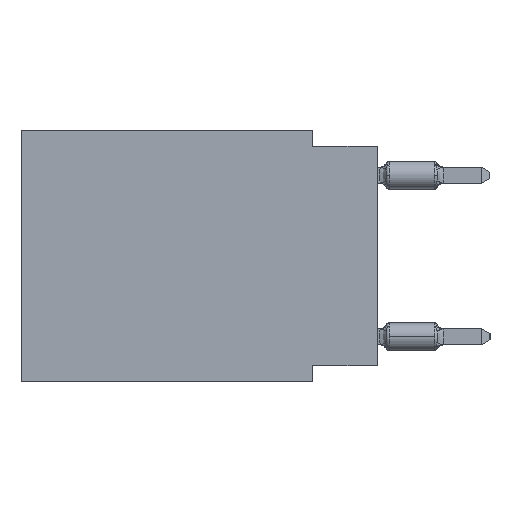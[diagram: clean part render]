
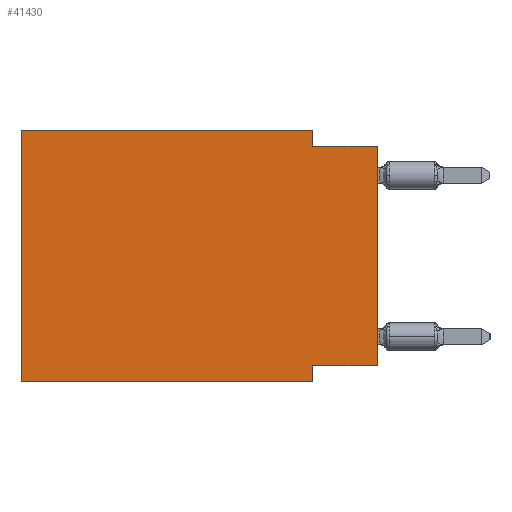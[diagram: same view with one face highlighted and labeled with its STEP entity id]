
A CAD part, left-side view. The second image highlights one B-rep face of the part: STEP entity #41430.
In plain terms, the highlighted planar face has unit normal (-1, 0, 0).
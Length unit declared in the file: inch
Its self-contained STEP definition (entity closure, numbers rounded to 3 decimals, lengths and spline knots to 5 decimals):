
#251 = EDGE_CURVE ( 'NONE', #14994, #14648, #38227, .T. ) ;
#1820 = EDGE_CURVE ( 'NONE', #37931, #29589, #4543, .T. ) ;
#2186 = DIRECTION ( 'NONE',  ( 0., 0., 1. ) ) ;
#2414 = CARTESIAN_POINT ( 'NONE',  ( 0., 0., 0. ) ) ;
#3234 = CARTESIAN_POINT ( 'NONE',  ( 0., 0.55, -0.39 ) ) ;
#4543 = LINE ( 'NONE', #5218, #20845 ) ;
#5218 = CARTESIAN_POINT ( 'NONE',  ( 0., 0.1, 0. ) ) ;
#6077 = DIRECTION ( 'NONE',  ( 0., 0., -1. ) ) ;
#8016 = ORIENTED_EDGE ( 'NONE', *, *, #33502, .T. ) ;
#8417 = CARTESIAN_POINT ( 'NONE',  ( 0., 0.1, -0.365 ) ) ;
#10371 = VERTEX_POINT ( 'NONE', #8417 ) ;
#11001 = ORIENTED_EDGE ( 'NONE', *, *, #20388, .F. ) ;
#11477 = VECTOR ( 'NONE', #44151, 39.37008 ) ;
#11637 = DIRECTION ( 'NONE',  ( 0., 0., -1. ) ) ;
#11897 = EDGE_LOOP ( 'NONE', ( #8016, #33574, #43823, #37226, #11001, #32263, #31227, #36981 ) ) ;
#12938 = CARTESIAN_POINT ( 'NONE',  ( 0., 0.1, -0.39 ) ) ;
#14648 = VERTEX_POINT ( 'NONE', #43078 ) ;
#14994 = VERTEX_POINT ( 'NONE', #20592 ) ;
#15985 = VECTOR ( 'NONE', #43843, 39.37008 ) ;
#16177 = CARTESIAN_POINT ( 'NONE',  ( 0., 0.1, -0.025 ) ) ;
#16811 = FACE_OUTER_BOUND ( 'NONE', #11897, .T. ) ;
#17160 = DIRECTION ( 'NONE',  ( 0., -1., 0. ) ) ;
#17559 = LINE ( 'NONE', #31271, #32658 ) ;
#17664 = CARTESIAN_POINT ( 'NONE',  ( 0., 0., -0.365 ) ) ;
#20088 = EDGE_CURVE ( 'NONE', #29589, #35310, #26798, .T. ) ;
#20388 = EDGE_CURVE ( 'NONE', #14994, #23673, #39596, .T. ) ;
#20592 = CARTESIAN_POINT ( 'NONE',  ( 0., 0.55, -0.39 ) ) ;
#20845 = VECTOR ( 'NONE', #11637, 39.37008 ) ;
#21084 = LINE ( 'NONE', #42143, #21763 ) ;
#21737 = AXIS2_PLACEMENT_3D ( 'NONE', #23464, #27325, #6077 ) ;
#21763 = VECTOR ( 'NONE', #22000, 39.37008 ) ;
#21846 = CARTESIAN_POINT ( 'NONE',  ( 0., 0.1, 0. ) ) ;
#22000 = DIRECTION ( 'NONE',  ( 0., -1., 0. ) ) ;
#22215 = VERTEX_POINT ( 'NONE', #17664 ) ;
#23464 = CARTESIAN_POINT ( 'NONE',  ( 0., 0.55, 0. ) ) ;
#23673 = VERTEX_POINT ( 'NONE', #37090 ) ;
#24716 = EDGE_CURVE ( 'NONE', #10371, #14648, #41082, .T. ) ;
#26798 = LINE ( 'NONE', #30451, #45062 ) ;
#27325 = DIRECTION ( 'NONE',  ( 1., 0., 0. ) ) ;
#29589 = VERTEX_POINT ( 'NONE', #16177 ) ;
#29962 = VECTOR ( 'NONE', #2186, 39.37008 ) ;
#30451 = CARTESIAN_POINT ( 'NONE',  ( 0., 0., -0.025 ) ) ;
#31227 = ORIENTED_EDGE ( 'NONE', *, *, #24716, .F. ) ;
#31271 = CARTESIAN_POINT ( 'NONE',  ( 0., 0., -0.365 ) ) ;
#31445 = PLANE ( 'NONE',  #21737 ) ;
#32263 = ORIENTED_EDGE ( 'NONE', *, *, #251, .T. ) ;
#32512 = CARTESIAN_POINT ( 'NONE',  ( 0., 0., -0.025 ) ) ;
#32658 = VECTOR ( 'NONE', #34961, 39.37008 ) ;
#33502 = EDGE_CURVE ( 'NONE', #22215, #35310, #33735, .T. ) ;
#33574 = ORIENTED_EDGE ( 'NONE', *, *, #20088, .F. ) ;
#33735 = LINE ( 'NONE', #2414, #29962 ) ;
#34961 = DIRECTION ( 'NONE',  ( 0., 1., 0. ) ) ;
#35310 = VERTEX_POINT ( 'NONE', #32512 ) ;
#36981 = ORIENTED_EDGE ( 'NONE', *, *, #40906, .F. ) ;
#37090 = CARTESIAN_POINT ( 'NONE',  ( 0., 0.55, 0. ) ) ;
#37226 = ORIENTED_EDGE ( 'NONE', *, *, #43272, .F. ) ;
#37931 = VERTEX_POINT ( 'NONE', #21846 ) ;
#38227 = LINE ( 'NONE', #3234, #41947 ) ;
#39596 = LINE ( 'NONE', #41387, #11477 ) ;
#40906 = EDGE_CURVE ( 'NONE', #22215, #10371, #17559, .T. ) ;
#41082 = LINE ( 'NONE', #12938, #15985 ) ;
#41387 = CARTESIAN_POINT ( 'NONE',  ( 0., 0.55, 0. ) ) ;
#41430 = ADVANCED_FACE ( 'NONE', ( #16811 ), #31445, .F. ) ;
#41947 = VECTOR ( 'NONE', #17160, 39.37008 ) ;
#42143 = CARTESIAN_POINT ( 'NONE',  ( 0., 0.55, 0. ) ) ;
#43078 = CARTESIAN_POINT ( 'NONE',  ( 0., 0.1, -0.39 ) ) ;
#43272 = EDGE_CURVE ( 'NONE', #23673, #37931, #21084, .T. ) ;
#43823 = ORIENTED_EDGE ( 'NONE', *, *, #1820, .F. ) ;
#43843 = DIRECTION ( 'NONE',  ( 0., 0., -1. ) ) ;
#44151 = DIRECTION ( 'NONE',  ( 0., 0., 1. ) ) ;
#44432 = DIRECTION ( 'NONE',  ( 0., -1., 0. ) ) ;
#45062 = VECTOR ( 'NONE', #44432, 39.37008 ) ;
